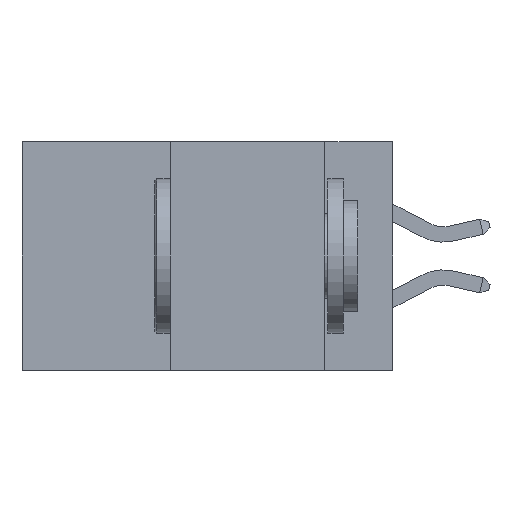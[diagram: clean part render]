
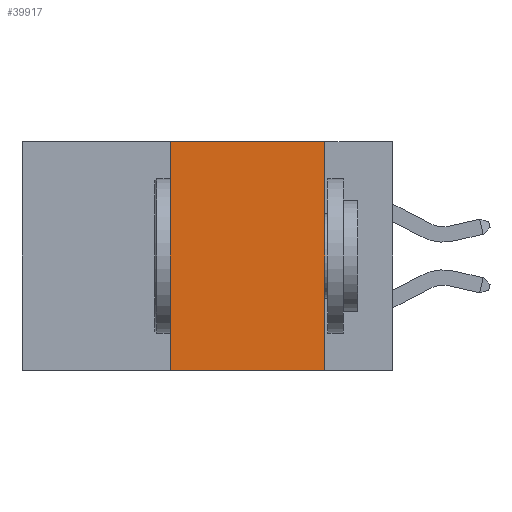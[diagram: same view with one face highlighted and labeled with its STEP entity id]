
A CAD part, left-side view. The second image highlights one B-rep face of the part: STEP entity #39917.
In plain terms, the highlighted planar face has unit normal (-1, 0, 0).
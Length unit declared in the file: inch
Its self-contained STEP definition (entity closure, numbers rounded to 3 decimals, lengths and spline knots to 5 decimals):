
#138 = VERTEX_POINT ( 'NONE', #35665 ) ;
#166 = DIRECTION ( 'NONE',  ( 0., -1., 0. ) ) ;
#309 = PLANE ( 'NONE',  #14500 ) ;
#396 = DIRECTION ( 'NONE',  ( 0., 0., 1. ) ) ;
#2651 = CARTESIAN_POINT ( 'NONE',  ( 0., 0.11, 0. ) ) ;
#3082 = VERTEX_POINT ( 'NONE', #11050 ) ;
#4631 = VERTEX_POINT ( 'NONE', #17783 ) ;
#6303 = LINE ( 'NONE', #25671, #13811 ) ;
#6746 = DIRECTION ( 'NONE',  ( 0., 0., -1. ) ) ;
#6921 = LINE ( 'NONE', #8662, #17440 ) ;
#8662 = CARTESIAN_POINT ( 'NONE',  ( 0., 0.6, -0.37 ) ) ;
#8879 = ORIENTED_EDGE ( 'NONE', *, *, #39889, .F. ) ;
#11050 = CARTESIAN_POINT ( 'NONE',  ( 0., 0.11, -0.37 ) ) ;
#13811 = VECTOR ( 'NONE', #166, 39.37008 ) ;
#14500 = AXIS2_PLACEMENT_3D ( 'NONE', #22741, #25965, #6746 ) ;
#15902 = ORIENTED_EDGE ( 'NONE', *, *, #23484, .T. ) ;
#17440 = VECTOR ( 'NONE', #34119, 39.37008 ) ;
#17783 = CARTESIAN_POINT ( 'NONE',  ( 0., 0.11, 0. ) ) ;
#20322 = VECTOR ( 'NONE', #28243, 39.37008 ) ;
#21327 = LINE ( 'NONE', #2651, #20322 ) ;
#22741 = CARTESIAN_POINT ( 'NONE',  ( 0., 0.6, 0. ) ) ;
#23420 = ORIENTED_EDGE ( 'NONE', *, *, #29852, .F. ) ;
#23484 = EDGE_CURVE ( 'NONE', #138, #3082, #6921, .T. ) ;
#25142 = LINE ( 'NONE', #38518, #31543 ) ;
#25671 = CARTESIAN_POINT ( 'NONE',  ( 0., 0.6, 0. ) ) ;
#25965 = DIRECTION ( 'NONE',  ( 1., 0., 0. ) ) ;
#28243 = DIRECTION ( 'NONE',  ( 0., 0., -1. ) ) ;
#28797 = FACE_OUTER_BOUND ( 'NONE', #35907, .T. ) ;
#29852 = EDGE_CURVE ( 'NONE', #138, #39935, #25142, .T. ) ;
#31299 = ORIENTED_EDGE ( 'NONE', *, *, #31961, .F. ) ;
#31543 = VECTOR ( 'NONE', #396, 39.37008 ) ;
#31961 = EDGE_CURVE ( 'NONE', #4631, #3082, #21327, .T. ) ;
#32267 = CARTESIAN_POINT ( 'NONE',  ( 0., 0.36, 0. ) ) ;
#34119 = DIRECTION ( 'NONE',  ( 0., -1., 0. ) ) ;
#35665 = CARTESIAN_POINT ( 'NONE',  ( 0., 0.36, -0.37 ) ) ;
#35907 = EDGE_LOOP ( 'NONE', ( #31299, #8879, #23420, #15902 ) ) ;
#38518 = CARTESIAN_POINT ( 'NONE',  ( 0., 0.36, 0. ) ) ;
#39889 = EDGE_CURVE ( 'NONE', #39935, #4631, #6303, .T. ) ;
#39917 = ADVANCED_FACE ( 'NONE', ( #28797 ), #309, .F. ) ;
#39935 = VERTEX_POINT ( 'NONE', #32267 ) ;
